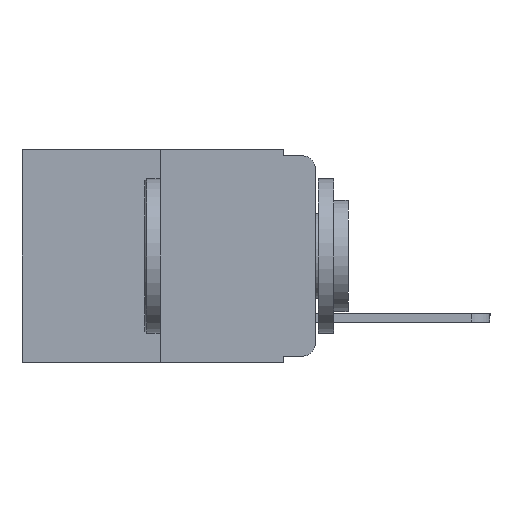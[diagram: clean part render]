
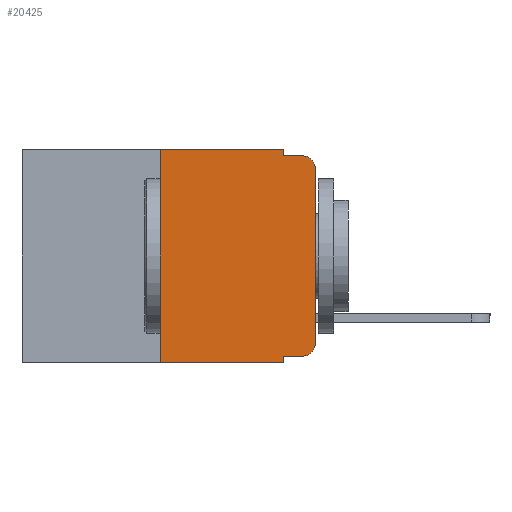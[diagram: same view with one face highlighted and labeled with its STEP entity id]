
A CAD part, left-side view. The second image highlights one B-rep face of the part: STEP entity #20425.
In plain terms, the highlighted planar face has unit normal (-1, 0, 0).
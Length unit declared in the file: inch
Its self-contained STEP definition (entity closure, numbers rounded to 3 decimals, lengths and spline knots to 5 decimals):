
#370 = DIRECTION ( 'NONE',  ( 0., 0., 1. ) ) ;
#532 = DIRECTION ( 'NONE',  ( 0., -1., 0. ) ) ;
#1133 = VECTOR ( 'NONE', #7457, 39.37008 ) ;
#1143 = CARTESIAN_POINT ( 'NONE',  ( 0., 0.051, -0.01 ) ) ;
#1306 = EDGE_CURVE ( 'NONE', #3451, #13206, #14064, .T. ) ;
#1498 = CARTESIAN_POINT ( 'NONE',  ( 0., 0.02, -0.333 ) ) ;
#1518 = CARTESIAN_POINT ( 'NONE',  ( 0., 0.051, -0.333 ) ) ;
#2408 = DIRECTION ( 'NONE',  ( 0., 0., 1. ) ) ;
#2563 = DIRECTION ( 'NONE',  ( 0., -1., 0. ) ) ;
#2572 = VECTOR ( 'NONE', #18524, 39.37008 ) ;
#2632 = CARTESIAN_POINT ( 'NONE',  ( 0., 0.051, 0. ) ) ;
#3282 = CARTESIAN_POINT ( 'NONE',  ( 0., 0.02, -0.313 ) ) ;
#3451 = VERTEX_POINT ( 'NONE', #18230 ) ;
#3530 = CARTESIAN_POINT ( 'NONE',  ( 0., 0.473, 0. ) ) ;
#3703 = ORIENTED_EDGE ( 'NONE', *, *, #8258, .F. ) ;
#3978 = VERTEX_POINT ( 'NONE', #5423 ) ;
#3994 = LINE ( 'NONE', #5928, #12820 ) ;
#4104 = CARTESIAN_POINT ( 'NONE',  ( 0., 0.473, -0.343 ) ) ;
#4135 = VECTOR ( 'NONE', #2408, 39.37008 ) ;
#4196 = EDGE_CURVE ( 'NONE', #12876, #12514, #22272, .T. ) ;
#4947 = VERTEX_POINT ( 'NONE', #14926 ) ;
#5129 = DIRECTION ( 'NONE',  ( 0., 0., -1. ) ) ;
#5223 = CIRCLE ( 'NONE', #15190, 0.02 ) ;
#5310 = FACE_OUTER_BOUND ( 'NONE', #17055, .T. ) ;
#5384 = DIRECTION ( 'NONE',  ( 0., 0., -1. ) ) ;
#5423 = CARTESIAN_POINT ( 'NONE',  ( 0., 0.051, -0.343 ) ) ;
#5675 = CARTESIAN_POINT ( 'NONE',  ( 0., 0.051, 0. ) ) ;
#5928 = CARTESIAN_POINT ( 'NONE',  ( 0., 0.473, 0. ) ) ;
#6434 = VERTEX_POINT ( 'NONE', #21970 ) ;
#7064 = EDGE_CURVE ( 'NONE', #10982, #18008, #9340, .T. ) ;
#7321 = VECTOR ( 'NONE', #370, 39.37008 ) ;
#7457 = DIRECTION ( 'NONE',  ( 0., 0., -1. ) ) ;
#7700 = DIRECTION ( 'NONE',  ( 0., -1., 0. ) ) ;
#7743 = CARTESIAN_POINT ( 'NONE',  ( 0., 0.051, -0.01 ) ) ;
#8204 = ORIENTED_EDGE ( 'NONE', *, *, #15291, .F. ) ;
#8258 = EDGE_CURVE ( 'NONE', #10982, #3978, #12556, .T. ) ;
#8458 = ORIENTED_EDGE ( 'NONE', *, *, #19517, .T. ) ;
#8731 = ORIENTED_EDGE ( 'NONE', *, *, #16397, .F. ) ;
#8851 = PLANE ( 'NONE',  #17517 ) ;
#9340 = LINE ( 'NONE', #11555, #18075 ) ;
#9557 = ORIENTED_EDGE ( 'NONE', *, *, #7064, .T. ) ;
#9894 = CARTESIAN_POINT ( 'NONE',  ( 0., 0.02, -0.03 ) ) ;
#10105 = ORIENTED_EDGE ( 'NONE', *, *, #17590, .F. ) ;
#10982 = VERTEX_POINT ( 'NONE', #1518 ) ;
#11347 = CIRCLE ( 'NONE', #20013, 0.02 ) ;
#11555 = CARTESIAN_POINT ( 'NONE',  ( 0., 0.051, -0.333 ) ) ;
#11611 = DIRECTION ( 'NONE',  ( 0., 0., -1. ) ) ;
#12514 = VERTEX_POINT ( 'NONE', #14399 ) ;
#12556 = LINE ( 'NONE', #2632, #2572 ) ;
#12820 = VECTOR ( 'NONE', #7700, 39.37008 ) ;
#12831 = CARTESIAN_POINT ( 'NONE',  ( 0., 0.25, 0. ) ) ;
#12876 = VERTEX_POINT ( 'NONE', #1143 ) ;
#13206 = VERTEX_POINT ( 'NONE', #17893 ) ;
#14064 = LINE ( 'NONE', #14614, #4135 ) ;
#14399 = CARTESIAN_POINT ( 'NONE',  ( 0., 0.02, -0.01 ) ) ;
#14614 = CARTESIAN_POINT ( 'NONE',  ( 0., 0., 0. ) ) ;
#14663 = EDGE_CURVE ( 'NONE', #19371, #3978, #17763, .T. ) ;
#14728 = ORIENTED_EDGE ( 'NONE', *, *, #22694, .T. ) ;
#14926 = CARTESIAN_POINT ( 'NONE',  ( 0., 0.25, 0. ) ) ;
#15190 = AXIS2_PLACEMENT_3D ( 'NONE', #3282, #15588, #5129 ) ;
#15291 = EDGE_CURVE ( 'NONE', #4947, #6434, #3994, .T. ) ;
#15526 = ORIENTED_EDGE ( 'NONE', *, *, #14663, .T. ) ;
#15588 = DIRECTION ( 'NONE',  ( -1., 0., 0. ) ) ;
#15798 = LINE ( 'NONE', #5675, #1133 ) ;
#15834 = DIRECTION ( 'NONE',  ( 1., 0., 0. ) ) ;
#16311 = DIRECTION ( 'NONE',  ( 0., -1., 0. ) ) ;
#16342 = CARTESIAN_POINT ( 'NONE',  ( 0., 0.25, -0.343 ) ) ;
#16397 = EDGE_CURVE ( 'NONE', #19371, #4947, #16580, .T. ) ;
#16580 = LINE ( 'NONE', #12831, #7321 ) ;
#17055 = EDGE_LOOP ( 'NONE', ( #21273, #8458, #17709, #10105, #8204, #8731, #15526, #3703, #9557, #14728 ) ) ;
#17080 = VECTOR ( 'NONE', #532, 39.37008 ) ;
#17228 = VECTOR ( 'NONE', #16311, 39.37008 ) ;
#17517 = AXIS2_PLACEMENT_3D ( 'NONE', #3530, #15834, #5384 ) ;
#17590 = EDGE_CURVE ( 'NONE', #6434, #12876, #15798, .T. ) ;
#17709 = ORIENTED_EDGE ( 'NONE', *, *, #4196, .F. ) ;
#17763 = LINE ( 'NONE', #4104, #17228 ) ;
#17893 = CARTESIAN_POINT ( 'NONE',  ( 0., 0., -0.03 ) ) ;
#18008 = VERTEX_POINT ( 'NONE', #1498 ) ;
#18075 = VECTOR ( 'NONE', #2563, 39.37008 ) ;
#18230 = CARTESIAN_POINT ( 'NONE',  ( 0., 0., -0.313 ) ) ;
#18524 = DIRECTION ( 'NONE',  ( 0., 0., -1. ) ) ;
#19371 = VERTEX_POINT ( 'NONE', #16342 ) ;
#19517 = EDGE_CURVE ( 'NONE', #13206, #12514, #11347, .T. ) ;
#20013 = AXIS2_PLACEMENT_3D ( 'NONE', #9894, #22082, #11611 ) ;
#20425 = ADVANCED_FACE ( 'NONE', ( #5310 ), #8851, .F. ) ;
#21273 = ORIENTED_EDGE ( 'NONE', *, *, #1306, .T. ) ;
#21970 = CARTESIAN_POINT ( 'NONE',  ( 0., 0.051, 0. ) ) ;
#22082 = DIRECTION ( 'NONE',  ( -1., 0., 0. ) ) ;
#22272 = LINE ( 'NONE', #7743, #17080 ) ;
#22694 = EDGE_CURVE ( 'NONE', #18008, #3451, #5223, .T. ) ;
